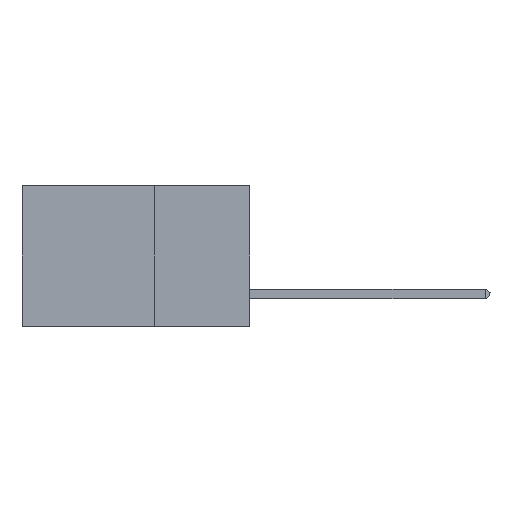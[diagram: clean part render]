
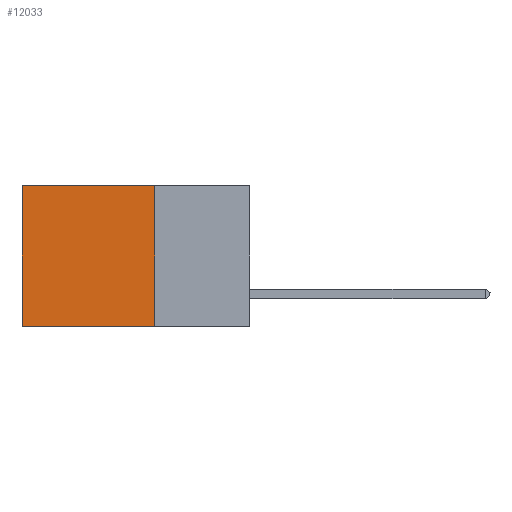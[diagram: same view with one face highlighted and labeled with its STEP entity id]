
A CAD part, left-side view. The second image highlights one B-rep face of the part: STEP entity #12033.
In plain terms, the highlighted planar face has unit normal (-1, 0, 0).
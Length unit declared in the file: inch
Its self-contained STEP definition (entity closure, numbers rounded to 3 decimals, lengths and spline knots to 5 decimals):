
#885 = LINE ( 'NONE', #17312, #29240 ) ;
#2894 = DIRECTION ( 'NONE',  ( 0., 1., 0. ) ) ;
#6634 = DIRECTION ( 'NONE',  ( 1., 0., 0. ) ) ;
#7322 = EDGE_CURVE ( 'NONE', #39049, #34942, #27601, .T. ) ;
#7370 = ORIENTED_EDGE ( 'NONE', *, *, #7322, .T. ) ;
#8616 = AXIS2_PLACEMENT_3D ( 'NONE', #33707, #6634, #41322 ) ;
#9293 = EDGE_CURVE ( 'NONE', #11929, #39049, #885, .T. ) ;
#11530 = EDGE_CURVE ( 'NONE', #11929, #35298, #45152, .T. ) ;
#11569 = ORIENTED_EDGE ( 'NONE', *, *, #45334, .F. ) ;
#11929 = VERTEX_POINT ( 'NONE', #36111 ) ;
#12033 = ADVANCED_FACE ( 'NONE', ( #37383 ), #14286, .F. ) ;
#14286 = PLANE ( 'NONE',  #8616 ) ;
#17312 = CARTESIAN_POINT ( 'NONE',  ( 0.2875, 0.25, 0. ) ) ;
#17584 = VECTOR ( 'NONE', #36199, 39.37008 ) ;
#18752 = DIRECTION ( 'NONE',  ( 0., 0., -1. ) ) ;
#20951 = CARTESIAN_POINT ( 'NONE',  ( 0.2875, 0.25, -0.37 ) ) ;
#21703 = CARTESIAN_POINT ( 'NONE',  ( 0.2875, 0.25, 0. ) ) ;
#22195 = ORIENTED_EDGE ( 'NONE', *, *, #9293, .T. ) ;
#25052 = VECTOR ( 'NONE', #29482, 39.37008 ) ;
#26505 = VECTOR ( 'NONE', #18752, 39.37008 ) ;
#27601 = LINE ( 'NONE', #33820, #26505 ) ;
#28106 = EDGE_LOOP ( 'NONE', ( #7370, #11569, #39680, #22195 ) ) ;
#28851 = CARTESIAN_POINT ( 'NONE',  ( 0.2875, 0.6, -0.37 ) ) ;
#29240 = VECTOR ( 'NONE', #2894, 39.37008 ) ;
#29482 = DIRECTION ( 'NONE',  ( 0., 1., 0. ) ) ;
#30544 = CARTESIAN_POINT ( 'NONE',  ( 0.2875, 0.6, 0. ) ) ;
#33707 = CARTESIAN_POINT ( 'NONE',  ( 0.2875, 0.25, 0. ) ) ;
#33820 = CARTESIAN_POINT ( 'NONE',  ( 0.2875, 0.6, 0. ) ) ;
#34942 = VERTEX_POINT ( 'NONE', #28851 ) ;
#35298 = VERTEX_POINT ( 'NONE', #20951 ) ;
#36111 = CARTESIAN_POINT ( 'NONE',  ( 0.2875, 0.25, 0. ) ) ;
#36199 = DIRECTION ( 'NONE',  ( 0., 0., -1. ) ) ;
#37383 = FACE_OUTER_BOUND ( 'NONE', #28106, .T. ) ;
#39049 = VERTEX_POINT ( 'NONE', #30544 ) ;
#39300 = LINE ( 'NONE', #44939, #25052 ) ;
#39680 = ORIENTED_EDGE ( 'NONE', *, *, #11530, .F. ) ;
#41322 = DIRECTION ( 'NONE',  ( 0., 0., -1. ) ) ;
#44939 = CARTESIAN_POINT ( 'NONE',  ( 0.2875, 0.25, -0.37 ) ) ;
#45152 = LINE ( 'NONE', #21703, #17584 ) ;
#45334 = EDGE_CURVE ( 'NONE', #35298, #34942, #39300, .T. ) ;
